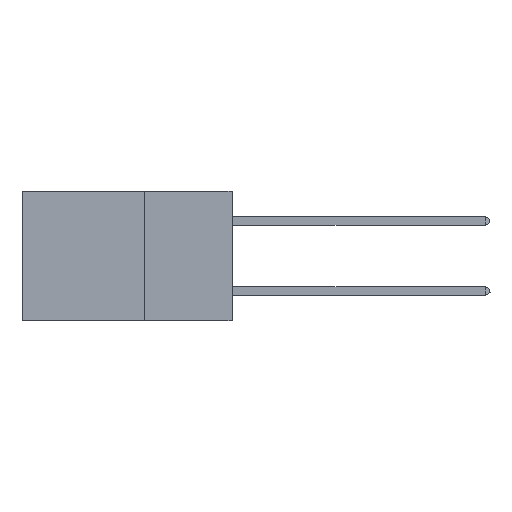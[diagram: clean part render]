
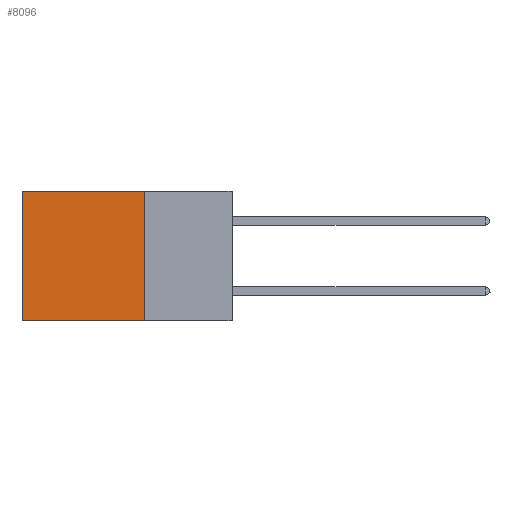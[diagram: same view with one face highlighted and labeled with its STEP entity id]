
A CAD part, left-side view. The second image highlights one B-rep face of the part: STEP entity #8096.
In plain terms, the highlighted planar face has unit normal (-1, 0, 0).
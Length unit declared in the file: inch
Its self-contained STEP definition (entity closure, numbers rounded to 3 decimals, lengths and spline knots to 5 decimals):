
#23 = VECTOR ( 'NONE', #12873, 39.37008 ) ;
#707 = CARTESIAN_POINT ( 'NONE',  ( 0.2875, 0.6, -0.37 ) ) ;
#1357 = VERTEX_POINT ( 'NONE', #8006 ) ;
#3798 = CARTESIAN_POINT ( 'NONE',  ( 0.2875, 0.25, -0.37 ) ) ;
#4306 = EDGE_CURVE ( 'NONE', #5397, #1357, #19999, .T. ) ;
#4491 = ORIENTED_EDGE ( 'NONE', *, *, #4306, .T. ) ;
#4722 = PLANE ( 'NONE',  #7872 ) ;
#4910 = CARTESIAN_POINT ( 'NONE',  ( 0.2875, 0.25, 0. ) ) ;
#5089 = CARTESIAN_POINT ( 'NONE',  ( 0.2875, 0.6, 0. ) ) ;
#5397 = VERTEX_POINT ( 'NONE', #31686 ) ;
#5727 = EDGE_CURVE ( 'NONE', #27937, #25720, #18356, .T. ) ;
#7872 = AXIS2_PLACEMENT_3D ( 'NONE', #24986, #12600, #25304 ) ;
#8006 = CARTESIAN_POINT ( 'NONE',  ( 0.2875, 0.6, 0. ) ) ;
#8096 = ADVANCED_FACE ( 'NONE', ( #29926 ), #4722, .F. ) ;
#10480 = CARTESIAN_POINT ( 'NONE',  ( 0.2875, 0.25, 0. ) ) ;
#11367 = EDGE_LOOP ( 'NONE', ( #23049, #16649, #12197, #4491 ) ) ;
#11940 = EDGE_CURVE ( 'NONE', #5397, #27937, #25831, .T. ) ;
#12197 = ORIENTED_EDGE ( 'NONE', *, *, #11940, .F. ) ;
#12600 = DIRECTION ( 'NONE',  ( 1., 0., 0. ) ) ;
#12873 = DIRECTION ( 'NONE',  ( 0., 0., -1. ) ) ;
#16649 = ORIENTED_EDGE ( 'NONE', *, *, #5727, .F. ) ;
#18356 = LINE ( 'NONE', #20569, #26236 ) ;
#19999 = LINE ( 'NONE', #10480, #20373 ) ;
#20373 = VECTOR ( 'NONE', #23183, 39.37008 ) ;
#20569 = CARTESIAN_POINT ( 'NONE',  ( 0.2875, 0.25, -0.37 ) ) ;
#22578 = EDGE_CURVE ( 'NONE', #1357, #25720, #25835, .T. ) ;
#23049 = ORIENTED_EDGE ( 'NONE', *, *, #22578, .T. ) ;
#23183 = DIRECTION ( 'NONE',  ( 0., 1., 0. ) ) ;
#24986 = CARTESIAN_POINT ( 'NONE',  ( 0.2875, 0.25, 0. ) ) ;
#25304 = DIRECTION ( 'NONE',  ( 0., 0., -1. ) ) ;
#25720 = VERTEX_POINT ( 'NONE', #707 ) ;
#25831 = LINE ( 'NONE', #4910, #26219 ) ;
#25835 = LINE ( 'NONE', #5089, #23 ) ;
#26219 = VECTOR ( 'NONE', #30522, 39.37008 ) ;
#26236 = VECTOR ( 'NONE', #28185, 39.37008 ) ;
#27937 = VERTEX_POINT ( 'NONE', #3798 ) ;
#28185 = DIRECTION ( 'NONE',  ( 0., 1., 0. ) ) ;
#29926 = FACE_OUTER_BOUND ( 'NONE', #11367, .T. ) ;
#30522 = DIRECTION ( 'NONE',  ( 0., 0., -1. ) ) ;
#31686 = CARTESIAN_POINT ( 'NONE',  ( 0.2875, 0.25, 0. ) ) ;
